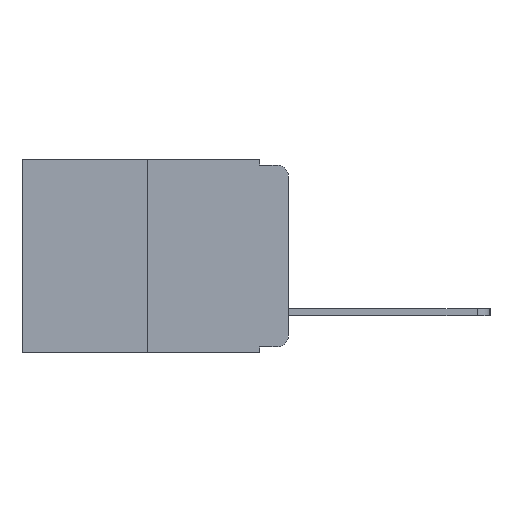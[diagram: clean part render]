
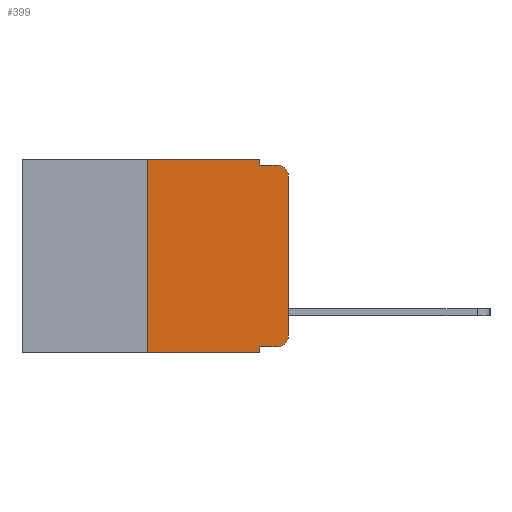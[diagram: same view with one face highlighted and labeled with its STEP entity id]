
A CAD part, left-side view. The second image highlights one B-rep face of the part: STEP entity #399.
In plain terms, the highlighted planar face has unit normal (-1, 0, 0).
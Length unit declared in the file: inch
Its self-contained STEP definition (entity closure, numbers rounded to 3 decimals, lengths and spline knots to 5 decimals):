
#208 = CARTESIAN_POINT ( 'NONE',  ( 0., 0.02, -0.03 ) ) ;
#304 = CARTESIAN_POINT ( 'NONE',  ( 0., 0.473, 0. ) ) ;
#399 = ADVANCED_FACE ( 'NONE', ( #8243 ), #10776, .F. ) ;
#524 = CARTESIAN_POINT ( 'NONE',  ( 0., 0.25, 0. ) ) ;
#531 = EDGE_CURVE ( 'NONE', #4868, #2564, #9548, .T. ) ;
#648 = LINE ( 'NONE', #524, #5388 ) ;
#697 = DIRECTION ( 'NONE',  ( 0., -1., 0. ) ) ;
#804 = CARTESIAN_POINT ( 'NONE',  ( 0., 0., 0. ) ) ;
#884 = CIRCLE ( 'NONE', #10966, 0.02 ) ;
#885 = CARTESIAN_POINT ( 'NONE',  ( 0., 0.051, -0.333 ) ) ;
#1033 = DIRECTION ( 'NONE',  ( 0., 0., 1. ) ) ;
#1195 = DIRECTION ( 'NONE',  ( 0., 0., -1. ) ) ;
#1260 = CIRCLE ( 'NONE', #4034, 0.02 ) ;
#1436 = EDGE_CURVE ( 'NONE', #8091, #4868, #884, .T. ) ;
#1872 = CARTESIAN_POINT ( 'NONE',  ( 0., 0.051, 0. ) ) ;
#1894 = DIRECTION ( 'NONE',  ( 0., 0., 1. ) ) ;
#2090 = LINE ( 'NONE', #304, #7574 ) ;
#2318 = VECTOR ( 'NONE', #1033, 39.37008 ) ;
#2503 = VERTEX_POINT ( 'NONE', #7734 ) ;
#2564 = VERTEX_POINT ( 'NONE', #5326 ) ;
#2689 = ORIENTED_EDGE ( 'NONE', *, *, #531, .T. ) ;
#3003 = ORIENTED_EDGE ( 'NONE', *, *, #6458, .F. ) ;
#3106 = VERTEX_POINT ( 'NONE', #9806 ) ;
#3165 = CARTESIAN_POINT ( 'NONE',  ( 0., 0.051, -0.01 ) ) ;
#3403 = EDGE_CURVE ( 'NONE', #8691, #8091, #8395, .T. ) ;
#3507 = EDGE_CURVE ( 'NONE', #8093, #8859, #11612, .T. ) ;
#3675 = VERTEX_POINT ( 'NONE', #1872 ) ;
#3862 = ORIENTED_EDGE ( 'NONE', *, *, #1436, .T. ) ;
#3887 = VECTOR ( 'NONE', #9445, 39.37008 ) ;
#4020 = EDGE_CURVE ( 'NONE', #8691, #8859, #7031, .T. ) ;
#4034 = AXIS2_PLACEMENT_3D ( 'NONE', #208, #6814, #1195 ) ;
#4056 = CARTESIAN_POINT ( 'NONE',  ( 0., 0.051, -0.343 ) ) ;
#4495 = EDGE_CURVE ( 'NONE', #2503, #3675, #2090, .T. ) ;
#4525 = LINE ( 'NONE', #5137, #11005 ) ;
#4584 = VECTOR ( 'NONE', #5931, 39.37008 ) ;
#4834 = CARTESIAN_POINT ( 'NONE',  ( 0., 0., -0.313 ) ) ;
#4868 = VERTEX_POINT ( 'NONE', #4834 ) ;
#5137 = CARTESIAN_POINT ( 'NONE',  ( 0., 0.051, 0. ) ) ;
#5151 = ORIENTED_EDGE ( 'NONE', *, *, #10551, .T. ) ;
#5245 = DIRECTION ( 'NONE',  ( 1., 0., 0. ) ) ;
#5326 = CARTESIAN_POINT ( 'NONE',  ( 0., 0., -0.03 ) ) ;
#5388 = VECTOR ( 'NONE', #1894, 39.37008 ) ;
#5423 = ORIENTED_EDGE ( 'NONE', *, *, #4495, .F. ) ;
#5729 = ORIENTED_EDGE ( 'NONE', *, *, #3507, .T. ) ;
#5750 = CARTESIAN_POINT ( 'NONE',  ( 0., 0.02, -0.333 ) ) ;
#5756 = VECTOR ( 'NONE', #8560, 39.37008 ) ;
#5862 = EDGE_CURVE ( 'NONE', #8093, #2503, #648, .T. ) ;
#5931 = DIRECTION ( 'NONE',  ( 0., 0., -1. ) ) ;
#6073 = DIRECTION ( 'NONE',  ( 0., 0., -1. ) ) ;
#6099 = CARTESIAN_POINT ( 'NONE',  ( 0., 0.051, 0. ) ) ;
#6458 = EDGE_CURVE ( 'NONE', #3675, #3106, #4525, .T. ) ;
#6657 = CARTESIAN_POINT ( 'NONE',  ( 0., 0.25, -0.343 ) ) ;
#6814 = DIRECTION ( 'NONE',  ( -1., 0., 0. ) ) ;
#7031 = LINE ( 'NONE', #6099, #4584 ) ;
#7383 = EDGE_LOOP ( 'NONE', ( #2689, #5151, #7573, #3003, #5423, #7852, #5729, #8109, #8369, #3862 ) ) ;
#7573 = ORIENTED_EDGE ( 'NONE', *, *, #7678, .F. ) ;
#7574 = VECTOR ( 'NONE', #697, 39.37008 ) ;
#7593 = AXIS2_PLACEMENT_3D ( 'NONE', #11363, #5245, #8913 ) ;
#7678 = EDGE_CURVE ( 'NONE', #3106, #10087, #10680, .T. ) ;
#7734 = CARTESIAN_POINT ( 'NONE',  ( 0., 0.25, 0. ) ) ;
#7852 = ORIENTED_EDGE ( 'NONE', *, *, #5862, .F. ) ;
#8091 = VERTEX_POINT ( 'NONE', #5750 ) ;
#8093 = VERTEX_POINT ( 'NONE', #6657 ) ;
#8109 = ORIENTED_EDGE ( 'NONE', *, *, #4020, .F. ) ;
#8243 = FACE_OUTER_BOUND ( 'NONE', #7383, .T. ) ;
#8354 = CARTESIAN_POINT ( 'NONE',  ( 0., 0.473, -0.343 ) ) ;
#8369 = ORIENTED_EDGE ( 'NONE', *, *, #3403, .T. ) ;
#8378 = DIRECTION ( 'NONE',  ( 0., -1., 0. ) ) ;
#8395 = LINE ( 'NONE', #9504, #5756 ) ;
#8560 = DIRECTION ( 'NONE',  ( 0., -1., 0. ) ) ;
#8691 = VERTEX_POINT ( 'NONE', #885 ) ;
#8859 = VERTEX_POINT ( 'NONE', #4056 ) ;
#8913 = DIRECTION ( 'NONE',  ( 0., 0., -1. ) ) ;
#9362 = VECTOR ( 'NONE', #8378, 39.37008 ) ;
#9445 = DIRECTION ( 'NONE',  ( 0., -1., 0. ) ) ;
#9504 = CARTESIAN_POINT ( 'NONE',  ( 0., 0.051, -0.333 ) ) ;
#9548 = LINE ( 'NONE', #804, #2318 ) ;
#9806 = CARTESIAN_POINT ( 'NONE',  ( 0., 0.051, -0.01 ) ) ;
#10087 = VERTEX_POINT ( 'NONE', #11160 ) ;
#10219 = CARTESIAN_POINT ( 'NONE',  ( 0., 0.02, -0.313 ) ) ;
#10341 = DIRECTION ( 'NONE',  ( -1., 0., 0. ) ) ;
#10395 = DIRECTION ( 'NONE',  ( 0., 0., -1. ) ) ;
#10551 = EDGE_CURVE ( 'NONE', #2564, #10087, #1260, .T. ) ;
#10680 = LINE ( 'NONE', #3165, #3887 ) ;
#10776 = PLANE ( 'NONE',  #7593 ) ;
#10966 = AXIS2_PLACEMENT_3D ( 'NONE', #10219, #10341, #10395 ) ;
#11005 = VECTOR ( 'NONE', #6073, 39.37008 ) ;
#11160 = CARTESIAN_POINT ( 'NONE',  ( 0., 0.02, -0.01 ) ) ;
#11363 = CARTESIAN_POINT ( 'NONE',  ( 0., 0.473, 0. ) ) ;
#11612 = LINE ( 'NONE', #8354, #9362 ) ;
